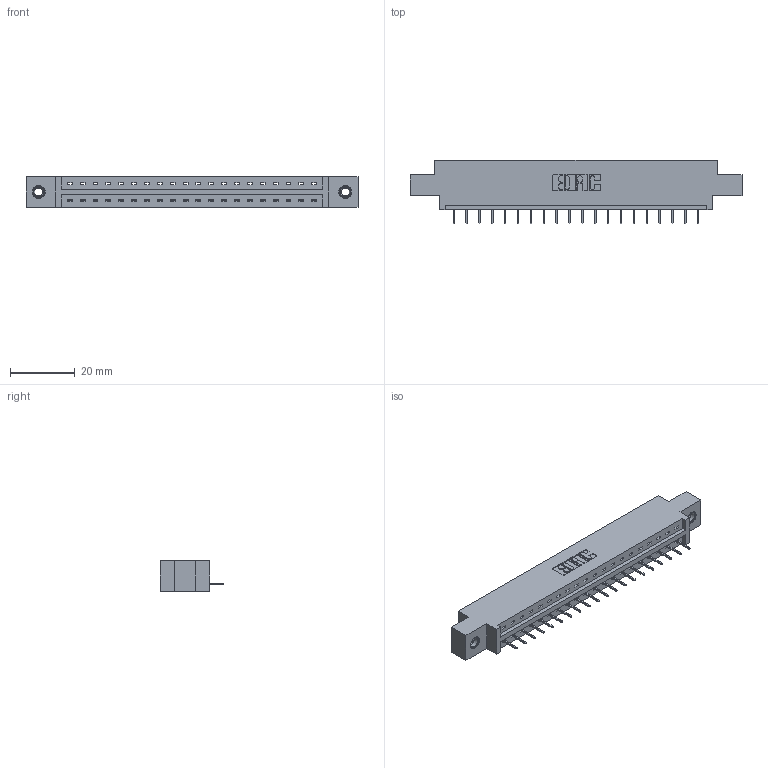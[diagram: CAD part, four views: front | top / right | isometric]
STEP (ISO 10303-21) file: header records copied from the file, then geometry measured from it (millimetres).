
FILE_DESCRIPTION (( 'STEP AP203' ), '1' );
FILE_NAME ('337-020-524-607.STEP', '2018-08-05T08:56:35', ( '' ), ( '' ), 'SwSTEP 2.0', 'SolidWorks 2016', '' );
FILE_SCHEMA (( 'CONFIG_CONTROL_DESIGN' ));
Length unit declared in the file: inch
Products named in the file (4): 337 Part_0.170 Offset - 0.156 Dia-TI; 345-292-001_345-293-124; 345-250-001_345-250-005-103; 337-020-524-607
Assembly tree (23 placements, depth 2):
  337-020-524-607
    337 Part_0.170 Offset - 0.156 Dia-TI
    345-292-001_345-293-124  x20
    345-250-001_345-250-005-103  x2
Bounding box: 102.26 x 19.69 x 9.4 mm (x, y, z)
Volume: 10142.9 mm3; surface area: 10218.7 mm2
Topology: 23 solids, 23 shells, 1498 faces, 4299 edges, 2778 vertices
Faces by surface type: plane 1146, cylinder 336, cone 12, torus 4
Entity records: 19104 total; most frequent: CARTESIAN_POINT 3305, ORIENTED_EDGE 3254, DIRECTION 2861, EDGE_CURVE 1627, VECTOR 1483, LINE 1483, VERTEX_POINT 1076, AXIS2_PLACEMENT_3D 689
